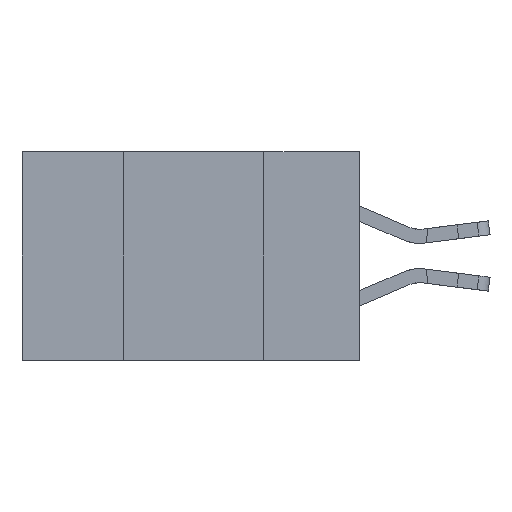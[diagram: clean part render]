
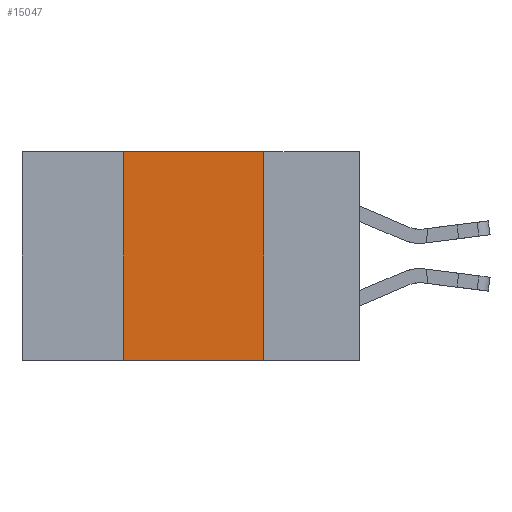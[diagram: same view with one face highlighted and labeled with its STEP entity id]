
A CAD part, left-side view. The second image highlights one B-rep face of the part: STEP entity #15047.
In plain terms, the highlighted planar face has unit normal (-1, 0, 0).
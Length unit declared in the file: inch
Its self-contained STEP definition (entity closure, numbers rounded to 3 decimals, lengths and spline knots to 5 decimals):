
#405 = CARTESIAN_POINT ( 'NONE',  ( 0., 0.42, -0.37 ) ) ;
#1593 = DIRECTION ( 'NONE',  ( 0., -1., 0. ) ) ;
#2329 = AXIS2_PLACEMENT_3D ( 'NONE', #13639, #4643, #15545 ) ;
#2573 = ORIENTED_EDGE ( 'NONE', *, *, #18063, .F. ) ;
#2642 = LINE ( 'NONE', #11855, #19449 ) ;
#2826 = VECTOR ( 'NONE', #3552, 39.37008 ) ;
#2853 = PLANE ( 'NONE',  #2329 ) ;
#3552 = DIRECTION ( 'NONE',  ( 0., 0., -1. ) ) ;
#3785 = EDGE_CURVE ( 'NONE', #14486, #21722, #4810, .T. ) ;
#4114 = EDGE_CURVE ( 'NONE', #11611, #8282, #18688, .T. ) ;
#4476 = CARTESIAN_POINT ( 'NONE',  ( 0., 0.17, -0.37 ) ) ;
#4643 = DIRECTION ( 'NONE',  ( 1., 0., 0. ) ) ;
#4810 = LINE ( 'NONE', #7157, #18156 ) ;
#7157 = CARTESIAN_POINT ( 'NONE',  ( 0., 0.6, 0. ) ) ;
#7443 = ORIENTED_EDGE ( 'NONE', *, *, #7779, .F. ) ;
#7577 = ORIENTED_EDGE ( 'NONE', *, *, #3785, .F. ) ;
#7779 = EDGE_CURVE ( 'NONE', #21722, #8282, #17317, .T. ) ;
#8282 = VERTEX_POINT ( 'NONE', #4476 ) ;
#9028 = VECTOR ( 'NONE', #21749, 39.37008 ) ;
#11611 = VERTEX_POINT ( 'NONE', #405 ) ;
#11855 = CARTESIAN_POINT ( 'NONE',  ( 0., 0.42, 0. ) ) ;
#12216 = ORIENTED_EDGE ( 'NONE', *, *, #4114, .T. ) ;
#13006 = FACE_OUTER_BOUND ( 'NONE', #19499, .T. ) ;
#13639 = CARTESIAN_POINT ( 'NONE',  ( 0., 0.6, 0. ) ) ;
#13839 = DIRECTION ( 'NONE',  ( 0., 0., 1. ) ) ;
#14486 = VERTEX_POINT ( 'NONE', #17753 ) ;
#14712 = CARTESIAN_POINT ( 'NONE',  ( 0., 0.17, 0. ) ) ;
#15047 = ADVANCED_FACE ( 'NONE', ( #13006 ), #2853, .F. ) ;
#15545 = DIRECTION ( 'NONE',  ( 0., 0., -1. ) ) ;
#16257 = CARTESIAN_POINT ( 'NONE',  ( 0., 0.6, -0.37 ) ) ;
#17317 = LINE ( 'NONE', #14712, #2826 ) ;
#17753 = CARTESIAN_POINT ( 'NONE',  ( 0., 0.42, 0. ) ) ;
#18063 = EDGE_CURVE ( 'NONE', #11611, #14486, #2642, .T. ) ;
#18156 = VECTOR ( 'NONE', #1593, 39.37008 ) ;
#18688 = LINE ( 'NONE', #16257, #9028 ) ;
#19449 = VECTOR ( 'NONE', #13839, 39.37008 ) ;
#19499 = EDGE_LOOP ( 'NONE', ( #7443, #7577, #2573, #12216 ) ) ;
#21722 = VERTEX_POINT ( 'NONE', #22770 ) ;
#21749 = DIRECTION ( 'NONE',  ( 0., -1., 0. ) ) ;
#22770 = CARTESIAN_POINT ( 'NONE',  ( 0., 0.17, 0. ) ) ;
